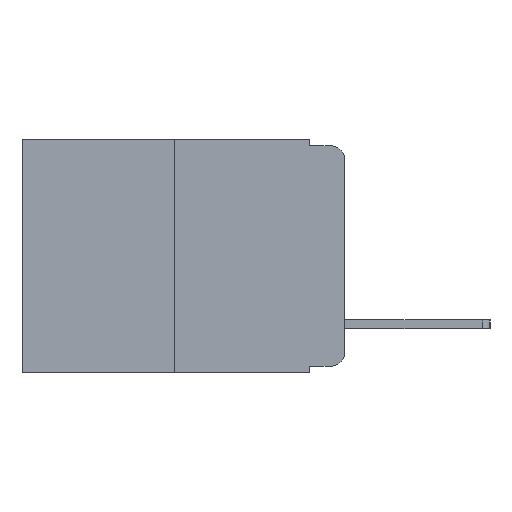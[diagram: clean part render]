
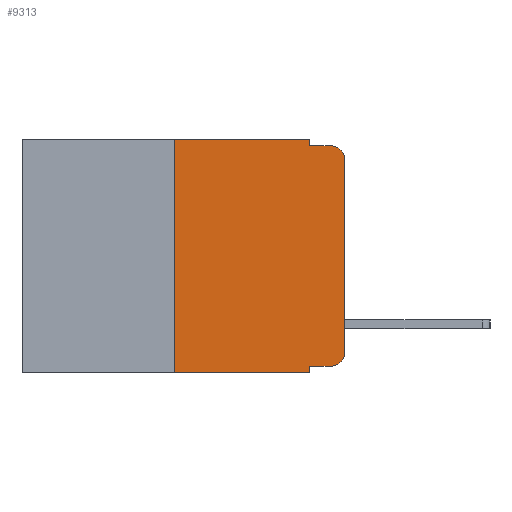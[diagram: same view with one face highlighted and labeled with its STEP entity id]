
A CAD part, left-side view. The second image highlights one B-rep face of the part: STEP entity #9313.
In plain terms, the highlighted planar face has unit normal (-1, 0, 0).
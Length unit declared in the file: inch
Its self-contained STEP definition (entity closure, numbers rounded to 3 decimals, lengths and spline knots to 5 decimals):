
#19 = EDGE_CURVE ( 'NONE', #18654, #13349, #14496, .T. ) ;
#334 = CARTESIAN_POINT ( 'NONE',  ( 0., 0.051, 0. ) ) ;
#688 = VERTEX_POINT ( 'NONE', #15260 ) ;
#1177 = EDGE_CURVE ( 'NONE', #688, #1797, #17216, .T. ) ;
#1562 = CARTESIAN_POINT ( 'NONE',  ( 0., 0.25, -0.343 ) ) ;
#1564 = CARTESIAN_POINT ( 'NONE',  ( 0., 0., -0.03 ) ) ;
#1626 = ORIENTED_EDGE ( 'NONE', *, *, #2235, .T. ) ;
#1631 = ORIENTED_EDGE ( 'NONE', *, *, #1177, .T. ) ;
#1797 = VERTEX_POINT ( 'NONE', #3281 ) ;
#1861 = ORIENTED_EDGE ( 'NONE', *, *, #8205, .F. ) ;
#2017 = ORIENTED_EDGE ( 'NONE', *, *, #19, .T. ) ;
#2046 = DIRECTION ( 'NONE',  ( 0., 0., -1. ) ) ;
#2088 = ORIENTED_EDGE ( 'NONE', *, *, #11233, .F. ) ;
#2235 = EDGE_CURVE ( 'NONE', #1797, #14724, #7945, .T. ) ;
#2263 = ORIENTED_EDGE ( 'NONE', *, *, #14674, .F. ) ;
#2556 = DIRECTION ( 'NONE',  ( 0., -1., 0. ) ) ;
#2958 = ORIENTED_EDGE ( 'NONE', *, *, #18302, .T. ) ;
#3281 = CARTESIAN_POINT ( 'NONE',  ( 0., 0.02, -0.333 ) ) ;
#3320 = AXIS2_PLACEMENT_3D ( 'NONE', #18543, #8565, #2046 ) ;
#3509 = CARTESIAN_POINT ( 'NONE',  ( 0., 0.473, 0. ) ) ;
#3732 = ORIENTED_EDGE ( 'NONE', *, *, #10792, .T. ) ;
#4207 = AXIS2_PLACEMENT_3D ( 'NONE', #18286, #19333, #11260 ) ;
#4492 = VERTEX_POINT ( 'NONE', #1564 ) ;
#4497 = CARTESIAN_POINT ( 'NONE',  ( 0., 0.051, 0. ) ) ;
#4949 = CARTESIAN_POINT ( 'NONE',  ( 0., 0.473, -0.343 ) ) ;
#5076 = LINE ( 'NONE', #18231, #9294 ) ;
#5439 = ORIENTED_EDGE ( 'NONE', *, *, #15471, .F. ) ;
#5716 = VERTEX_POINT ( 'NONE', #7814 ) ;
#5794 = VECTOR ( 'NONE', #2556, 39.37008 ) ;
#5939 = VECTOR ( 'NONE', #17609, 39.37008 ) ;
#6302 = ORIENTED_EDGE ( 'NONE', *, *, #6640, .F. ) ;
#6410 = VECTOR ( 'NONE', #11967, 39.37008 ) ;
#6640 = EDGE_CURVE ( 'NONE', #10961, #6920, #5076, .T. ) ;
#6717 = CARTESIAN_POINT ( 'NONE',  ( 0., 0.02, -0.03 ) ) ;
#6920 = VERTEX_POINT ( 'NONE', #17984 ) ;
#7370 = CARTESIAN_POINT ( 'NONE',  ( 0., 0.051, -0.343 ) ) ;
#7814 = CARTESIAN_POINT ( 'NONE',  ( 0., 0.25, 0. ) ) ;
#7945 = CIRCLE ( 'NONE', #3320, 0.02 ) ;
#8205 = EDGE_CURVE ( 'NONE', #688, #13349, #16813, .T. ) ;
#8290 = PLANE ( 'NONE',  #4207 ) ;
#8318 = DIRECTION ( 'NONE',  ( 0., 0., -1. ) ) ;
#8565 = DIRECTION ( 'NONE',  ( -1., 0., 0. ) ) ;
#9025 = CARTESIAN_POINT ( 'NONE',  ( 0., 0.02, -0.01 ) ) ;
#9125 = CIRCLE ( 'NONE', #17718, 0.02 ) ;
#9294 = VECTOR ( 'NONE', #15403, 39.37008 ) ;
#9313 = ADVANCED_FACE ( 'NONE', ( #14994 ), #8290, .F. ) ;
#9712 = VECTOR ( 'NONE', #14962, 39.37008 ) ;
#9766 = VECTOR ( 'NONE', #16946, 39.37008 ) ;
#9965 = LINE ( 'NONE', #13261, #5794 ) ;
#10554 = LINE ( 'NONE', #13404, #5939 ) ;
#10710 = VECTOR ( 'NONE', #11101, 39.37008 ) ;
#10792 = EDGE_CURVE ( 'NONE', #4492, #16349, #9125, .T. ) ;
#10961 = VERTEX_POINT ( 'NONE', #334 ) ;
#11101 = DIRECTION ( 'NONE',  ( 0., -1., 0. ) ) ;
#11153 = DIRECTION ( 'NONE',  ( 0., -1., 0. ) ) ;
#11201 = CARTESIAN_POINT ( 'NONE',  ( 0., 0.051, -0.333 ) ) ;
#11233 = EDGE_CURVE ( 'NONE', #18654, #5716, #17575, .T. ) ;
#11260 = DIRECTION ( 'NONE',  ( 0., 0., -1. ) ) ;
#11967 = DIRECTION ( 'NONE',  ( 0., 0., 1. ) ) ;
#13261 = CARTESIAN_POINT ( 'NONE',  ( 0., 0.051, -0.01 ) ) ;
#13349 = VERTEX_POINT ( 'NONE', #7370 ) ;
#13404 = CARTESIAN_POINT ( 'NONE',  ( 0., 0., 0. ) ) ;
#13601 = LINE ( 'NONE', #3509, #9766 ) ;
#14198 = CARTESIAN_POINT ( 'NONE',  ( 0., 0., -0.313 ) ) ;
#14496 = LINE ( 'NONE', #4949, #10710 ) ;
#14674 = EDGE_CURVE ( 'NONE', #5716, #10961, #13601, .T. ) ;
#14724 = VERTEX_POINT ( 'NONE', #14198 ) ;
#14801 = CARTESIAN_POINT ( 'NONE',  ( 0., 0.25, 0. ) ) ;
#14962 = DIRECTION ( 'NONE',  ( 0., 0., -1. ) ) ;
#14994 = FACE_OUTER_BOUND ( 'NONE', #17994, .T. ) ;
#15260 = CARTESIAN_POINT ( 'NONE',  ( 0., 0.051, -0.333 ) ) ;
#15403 = DIRECTION ( 'NONE',  ( 0., 0., -1. ) ) ;
#15471 = EDGE_CURVE ( 'NONE', #6920, #16349, #9965, .T. ) ;
#16349 = VERTEX_POINT ( 'NONE', #9025 ) ;
#16813 = LINE ( 'NONE', #4497, #9712 ) ;
#16902 = DIRECTION ( 'NONE',  ( -1., 0., 0. ) ) ;
#16946 = DIRECTION ( 'NONE',  ( 0., -1., 0. ) ) ;
#17216 = LINE ( 'NONE', #11201, #17658 ) ;
#17575 = LINE ( 'NONE', #14801, #6410 ) ;
#17609 = DIRECTION ( 'NONE',  ( 0., 0., 1. ) ) ;
#17658 = VECTOR ( 'NONE', #11153, 39.37008 ) ;
#17718 = AXIS2_PLACEMENT_3D ( 'NONE', #6717, #16902, #8318 ) ;
#17984 = CARTESIAN_POINT ( 'NONE',  ( 0., 0.051, -0.01 ) ) ;
#17994 = EDGE_LOOP ( 'NONE', ( #2958, #3732, #5439, #6302, #2263, #2088, #2017, #1861, #1631, #1626 ) ) ;
#18231 = CARTESIAN_POINT ( 'NONE',  ( 0., 0.051, 0. ) ) ;
#18286 = CARTESIAN_POINT ( 'NONE',  ( 0., 0.473, 0. ) ) ;
#18302 = EDGE_CURVE ( 'NONE', #14724, #4492, #10554, .T. ) ;
#18543 = CARTESIAN_POINT ( 'NONE',  ( 0., 0.02, -0.313 ) ) ;
#18654 = VERTEX_POINT ( 'NONE', #1562 ) ;
#19333 = DIRECTION ( 'NONE',  ( 1., 0., 0. ) ) ;
